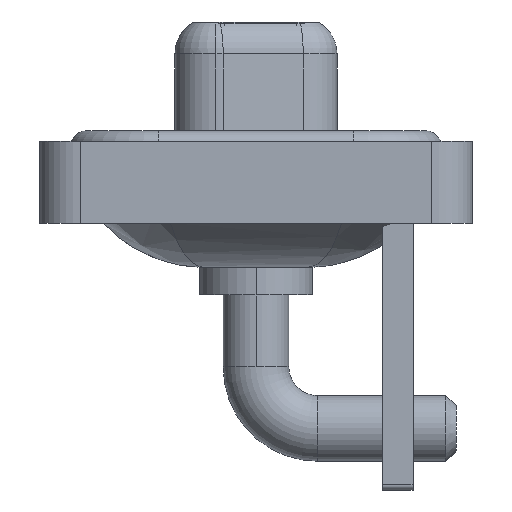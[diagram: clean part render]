
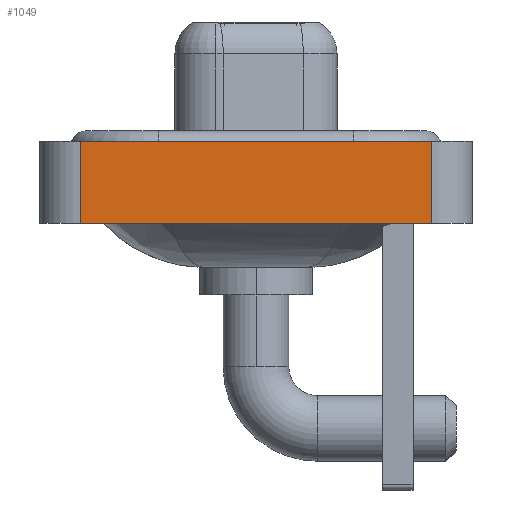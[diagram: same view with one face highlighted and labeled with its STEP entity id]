
A CAD part, left-side view. The second image highlights one B-rep face of the part: STEP entity #1049.
In plain terms, the highlighted planar face has unit normal (-1, 0, 0).
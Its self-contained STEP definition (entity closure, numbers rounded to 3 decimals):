
#524 = VECTOR ( 'NONE', #7636, 1000. ) ;
#589 = VECTOR ( 'NONE', #10814, 1000. ) ;
#714 = CARTESIAN_POINT ( 'NONE',  ( -7.25, -8.55, -3.6 ) ) ;
#1049 = ADVANCED_FACE ( 'NONE', ( #14850 ), #3580, .T. ) ;
#1797 = ORIENTED_EDGE ( 'NONE', *, *, #3875, .T. ) ;
#2032 = EDGE_CURVE ( 'NONE', #10151, #3424, #5524, .T. ) ;
#2221 = EDGE_CURVE ( 'NONE', #11801, #15160, #12230, .T. ) ;
#2676 = ORIENTED_EDGE ( 'NONE', *, *, #2032, .T. ) ;
#3022 = DIRECTION ( 'NONE',  ( 0., -1., 0. ) ) ;
#3267 = CARTESIAN_POINT ( 'NONE',  ( -7.25, -8.55, 0.4 ) ) ;
#3424 = VERTEX_POINT ( 'NONE', #11411 ) ;
#3537 = VECTOR ( 'NONE', #3022, 1000. ) ;
#3580 = PLANE ( 'NONE',  #8907 ) ;
#3875 = EDGE_CURVE ( 'NONE', #3424, #15160, #11392, .T. ) ;
#5524 = LINE ( 'NONE', #8058, #3537 ) ;
#6424 = EDGE_CURVE ( 'NONE', #10151, #11801, #8371, .T. ) ;
#6504 = CARTESIAN_POINT ( 'NONE',  ( -7.25, -8.55, 0.4 ) ) ;
#7636 = DIRECTION ( 'NONE',  ( 0., 0., 1. ) ) ;
#8058 = CARTESIAN_POINT ( 'NONE',  ( -7.25, -8.55, -3.6 ) ) ;
#8361 = DIRECTION ( 'NONE',  ( 0., 0., 1. ) ) ;
#8371 = LINE ( 'NONE', #13581, #15516 ) ;
#8907 = AXIS2_PLACEMENT_3D ( 'NONE', #714, #10949, #8361 ) ;
#10151 = VERTEX_POINT ( 'NONE', #15427 ) ;
#10158 = EDGE_LOOP ( 'NONE', ( #1797, #13713, #12663, #2676 ) ) ;
#10814 = DIRECTION ( 'NONE',  ( 0., -1., 0. ) ) ;
#10949 = DIRECTION ( 'NONE',  ( -1., 0., 0. ) ) ;
#11392 = LINE ( 'NONE', #14026, #524 ) ;
#11411 = CARTESIAN_POINT ( 'NONE',  ( -7.25, -8.55, -3.6 ) ) ;
#11801 = VERTEX_POINT ( 'NONE', #12912 ) ;
#12230 = LINE ( 'NONE', #3267, #589 ) ;
#12663 = ORIENTED_EDGE ( 'NONE', *, *, #6424, .F. ) ;
#12912 = CARTESIAN_POINT ( 'NONE',  ( -7.25, 8.55, 0.4 ) ) ;
#13502 = DIRECTION ( 'NONE',  ( 0., 0., 1. ) ) ;
#13581 = CARTESIAN_POINT ( 'NONE',  ( -7.25, 8.55, -3.6 ) ) ;
#13713 = ORIENTED_EDGE ( 'NONE', *, *, #2221, .F. ) ;
#14026 = CARTESIAN_POINT ( 'NONE',  ( -7.25, -8.55, -3.6 ) ) ;
#14850 = FACE_OUTER_BOUND ( 'NONE', #10158, .T. ) ;
#15160 = VERTEX_POINT ( 'NONE', #6504 ) ;
#15427 = CARTESIAN_POINT ( 'NONE',  ( -7.25, 8.55, -3.6 ) ) ;
#15516 = VECTOR ( 'NONE', #13502, 1000. ) ;
